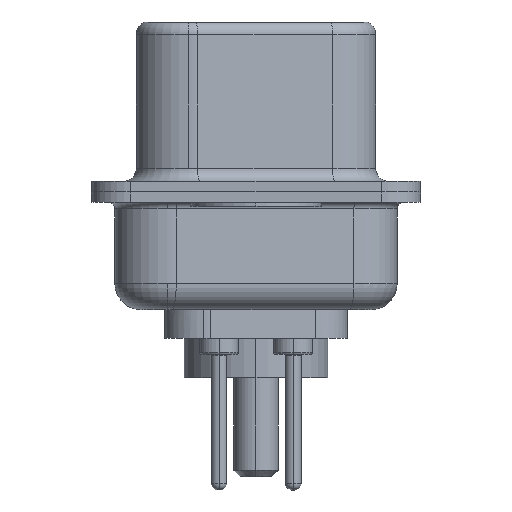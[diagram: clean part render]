
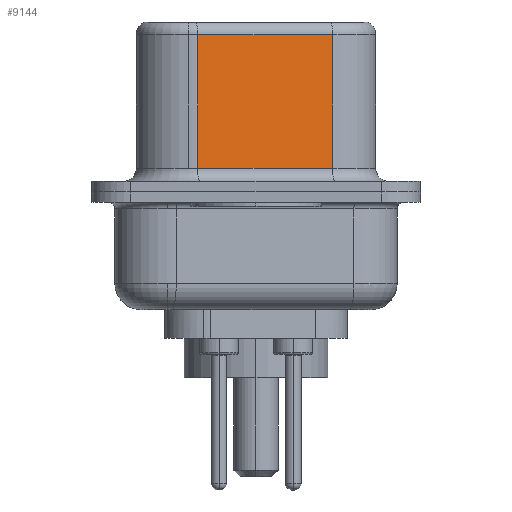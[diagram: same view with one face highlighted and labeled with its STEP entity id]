
A CAD part, left-side view. The second image highlights one B-rep face of the part: STEP entity #9144.
In plain terms, the highlighted planar face has unit normal (-0.985, -0.174, 0).
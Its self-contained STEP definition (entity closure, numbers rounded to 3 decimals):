
#700 = PLANE ( 'NONE',  #8003 ) ;
#1164 = VECTOR ( 'NONE', #8163, 1000. ) ;
#1370 = EDGE_CURVE ( 'NONE', #8494, #8300, #5771, .T. ) ;
#1438 = EDGE_CURVE ( 'NONE', #11920, #8300, #7453, .T. ) ;
#1532 = LINE ( 'NONE', #13123, #1164 ) ;
#1643 = FACE_OUTER_BOUND ( 'NONE', #2166, .T. ) ;
#2012 = ORIENTED_EDGE ( 'NONE', *, *, #8890, .T. ) ;
#2166 = EDGE_LOOP ( 'NONE', ( #11451, #12143, #2012, #3325 ) ) ;
#2339 = CARTESIAN_POINT ( 'NONE',  ( 4.565, -2.927, 6.52 ) ) ;
#2641 = CARTESIAN_POINT ( 'NONE',  ( 3.655, 2.233, 6.52 ) ) ;
#3049 = DIRECTION ( 'NONE',  ( -0.174, 0.985, 0. ) ) ;
#3325 = ORIENTED_EDGE ( 'NONE', *, *, #1438, .T. ) ;
#3394 = DIRECTION ( 'NONE',  ( 0.174, -0.985, 0. ) ) ;
#3869 = CARTESIAN_POINT ( 'NONE',  ( 4.565, -2.927, 0.9 ) ) ;
#4506 = VECTOR ( 'NONE', #3394, 1000. ) ;
#5771 = LINE ( 'NONE', #2339, #8573 ) ;
#6290 = EDGE_CURVE ( 'NONE', #8494, #6674, #1532, .T. ) ;
#6532 = CARTESIAN_POINT ( 'NONE',  ( 4.565, -2.927, 6.52 ) ) ;
#6674 = VERTEX_POINT ( 'NONE', #14621 ) ;
#7398 = CARTESIAN_POINT ( 'NONE',  ( 3.655, 2.233, 0.9 ) ) ;
#7453 = LINE ( 'NONE', #10856, #4506 ) ;
#7940 = DIRECTION ( 'NONE',  ( 0., 0., -1. ) ) ;
#8003 = AXIS2_PLACEMENT_3D ( 'NONE', #6532, #10130, #3049 ) ;
#8163 = DIRECTION ( 'NONE',  ( -0.174, 0.985, 0. ) ) ;
#8300 = VERTEX_POINT ( 'NONE', #3869 ) ;
#8494 = VERTEX_POINT ( 'NONE', #15059 ) ;
#8573 = VECTOR ( 'NONE', #7940, 1000. ) ;
#8890 = EDGE_CURVE ( 'NONE', #6674, #11920, #14360, .T. ) ;
#9144 = ADVANCED_FACE ( 'NONE', ( #1643 ), #700, .F. ) ;
#9720 = DIRECTION ( 'NONE',  ( 0., 0., -1. ) ) ;
#10130 = DIRECTION ( 'NONE',  ( 0.985, 0.174, 0. ) ) ;
#10856 = CARTESIAN_POINT ( 'NONE',  ( 4.565, -2.927, 0.9 ) ) ;
#10869 = VECTOR ( 'NONE', #9720, 1000. ) ;
#11451 = ORIENTED_EDGE ( 'NONE', *, *, #1370, .F. ) ;
#11920 = VERTEX_POINT ( 'NONE', #7398 ) ;
#12143 = ORIENTED_EDGE ( 'NONE', *, *, #6290, .T. ) ;
#13123 = CARTESIAN_POINT ( 'NONE',  ( 4.565, -2.927, 6.02 ) ) ;
#14360 = LINE ( 'NONE', #2641, #10869 ) ;
#14621 = CARTESIAN_POINT ( 'NONE',  ( 3.655, 2.233, 6.02 ) ) ;
#15059 = CARTESIAN_POINT ( 'NONE',  ( 4.565, -2.927, 6.02 ) ) ;
